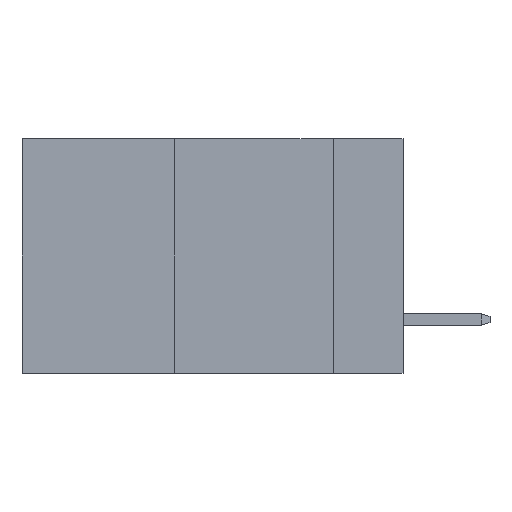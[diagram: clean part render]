
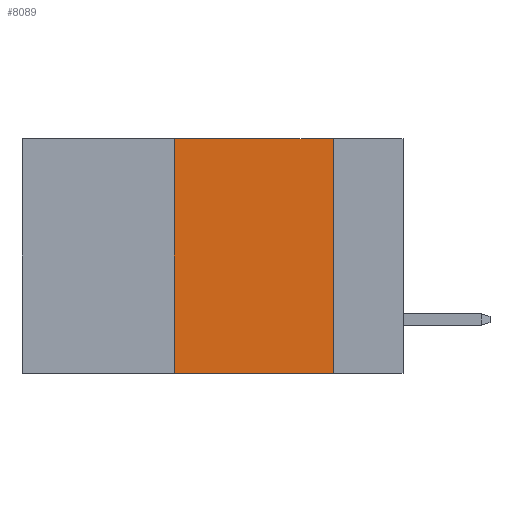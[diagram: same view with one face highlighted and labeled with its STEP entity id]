
A CAD part, left-side view. The second image highlights one B-rep face of the part: STEP entity #8089.
In plain terms, the highlighted planar face has unit normal (-1, 0, 0).
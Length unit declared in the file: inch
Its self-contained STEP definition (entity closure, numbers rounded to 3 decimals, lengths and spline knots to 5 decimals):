
#308 = VECTOR ( 'NONE', #11503, 39.37008 ) ;
#536 = AXIS2_PLACEMENT_3D ( 'NONE', #14093, #579, #13889 ) ;
#579 = DIRECTION ( 'NONE',  ( 1., 0., 0. ) ) ;
#1917 = VERTEX_POINT ( 'NONE', #12773 ) ;
#2035 = CARTESIAN_POINT ( 'NONE',  ( 0., 0.11, 0. ) ) ;
#2703 = CARTESIAN_POINT ( 'NONE',  ( 0., 0.11, 0. ) ) ;
#4374 = DIRECTION ( 'NONE',  ( 0., -1., 0. ) ) ;
#4632 = VERTEX_POINT ( 'NONE', #14486 ) ;
#4814 = VECTOR ( 'NONE', #11517, 39.37008 ) ;
#5031 = DIRECTION ( 'NONE',  ( 0., 0., 1. ) ) ;
#5529 = LINE ( 'NONE', #11110, #11775 ) ;
#6047 = VECTOR ( 'NONE', #5031, 39.37008 ) ;
#7369 = LINE ( 'NONE', #14127, #6047 ) ;
#7445 = EDGE_CURVE ( 'NONE', #4632, #11004, #5529, .T. ) ;
#7788 = CARTESIAN_POINT ( 'NONE',  ( 0., 0.11, -0.37 ) ) ;
#7819 = ORIENTED_EDGE ( 'NONE', *, *, #8403, .T. ) ;
#7837 = CARTESIAN_POINT ( 'NONE',  ( 0., 0.6, -0.37 ) ) ;
#7922 = VERTEX_POINT ( 'NONE', #7788 ) ;
#8089 = ADVANCED_FACE ( 'NONE', ( #8508 ), #9458, .F. ) ;
#8403 = EDGE_CURVE ( 'NONE', #1917, #7922, #13592, .T. ) ;
#8508 = FACE_OUTER_BOUND ( 'NONE', #11158, .T. ) ;
#9458 = PLANE ( 'NONE',  #536 ) ;
#9785 = ORIENTED_EDGE ( 'NONE', *, *, #12909, .F. ) ;
#10664 = EDGE_CURVE ( 'NONE', #11004, #7922, #12641, .T. ) ;
#11004 = VERTEX_POINT ( 'NONE', #2035 ) ;
#11064 = ORIENTED_EDGE ( 'NONE', *, *, #7445, .F. ) ;
#11110 = CARTESIAN_POINT ( 'NONE',  ( 0., 0.6, 0. ) ) ;
#11158 = EDGE_LOOP ( 'NONE', ( #12428, #11064, #9785, #7819 ) ) ;
#11503 = DIRECTION ( 'NONE',  ( 0., -1., 0. ) ) ;
#11517 = DIRECTION ( 'NONE',  ( 0., 0., -1. ) ) ;
#11775 = VECTOR ( 'NONE', #4374, 39.37008 ) ;
#12428 = ORIENTED_EDGE ( 'NONE', *, *, #10664, .F. ) ;
#12641 = LINE ( 'NONE', #2703, #4814 ) ;
#12773 = CARTESIAN_POINT ( 'NONE',  ( 0., 0.36, -0.37 ) ) ;
#12909 = EDGE_CURVE ( 'NONE', #1917, #4632, #7369, .T. ) ;
#13592 = LINE ( 'NONE', #7837, #308 ) ;
#13889 = DIRECTION ( 'NONE',  ( 0., 0., -1. ) ) ;
#14093 = CARTESIAN_POINT ( 'NONE',  ( 0., 0.6, 0. ) ) ;
#14127 = CARTESIAN_POINT ( 'NONE',  ( 0., 0.36, 0. ) ) ;
#14486 = CARTESIAN_POINT ( 'NONE',  ( 0., 0.36, 0. ) ) ;
